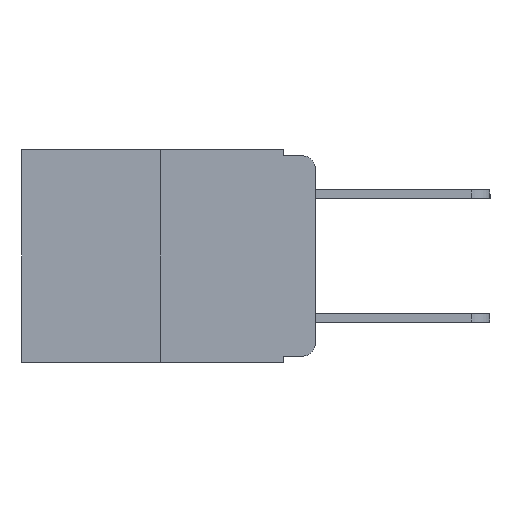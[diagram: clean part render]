
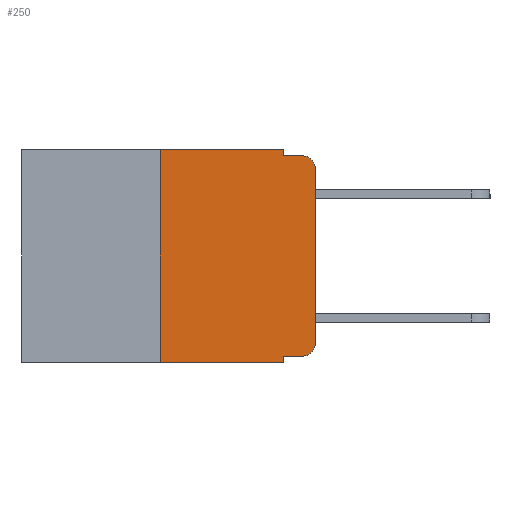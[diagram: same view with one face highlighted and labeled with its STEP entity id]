
A CAD part, left-side view. The second image highlights one B-rep face of the part: STEP entity #250.
In plain terms, the highlighted planar face has unit normal (-1, 0, 0).
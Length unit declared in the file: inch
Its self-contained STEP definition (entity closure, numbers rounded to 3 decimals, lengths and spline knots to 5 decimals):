
#221 = EDGE_CURVE ( 'NONE', #16890, #18291, #3032, .T. ) ;
#250 = ADVANCED_FACE ( 'NONE', ( #1961 ), #18845, .F. ) ;
#632 = EDGE_CURVE ( 'NONE', #7959, #7706, #19525, .T. ) ;
#660 = EDGE_CURVE ( 'NONE', #7706, #18892, #11691, .T. ) ;
#661 = EDGE_CURVE ( 'NONE', #12660, #18892, #18646, .T. ) ;
#666 = EDGE_CURVE ( 'NONE', #18397, #12660, #14743, .T. ) ;
#701 = EDGE_CURVE ( 'NONE', #16890, #14407, #1710, .T. ) ;
#729 = EDGE_CURVE ( 'NONE', #15698, #18291, #13327, .T. ) ;
#741 = EDGE_CURVE ( 'NONE', #15698, #6770, #8849, .T. ) ;
#771 = EDGE_CURVE ( 'NONE', #6770, #7959, #11453, .T. ) ;
#911 = DIRECTION ( 'NONE',  ( 0., 0., 1. ) ) ;
#1091 = CARTESIAN_POINT ( 'NONE',  ( 0., 0.473, 0. ) ) ;
#1710 = LINE ( 'NONE', #16748, #6252 ) ;
#1961 = FACE_OUTER_BOUND ( 'NONE', #14242, .T. ) ;
#2156 = DIRECTION ( 'NONE',  ( 0., -1., 0. ) ) ;
#2264 = DIRECTION ( 'NONE',  ( 0., 0., -1. ) ) ;
#2284 = VECTOR ( 'NONE', #2264, 39.37008 ) ;
#2516 = DIRECTION ( 'NONE',  ( 0., 0., -1. ) ) ;
#2539 = DIRECTION ( 'NONE',  ( 1., 0., 0. ) ) ;
#2591 = CARTESIAN_POINT ( 'NONE',  ( 0., 0.051, -0.01 ) ) ;
#2787 = CARTESIAN_POINT ( 'NONE',  ( 0., 0.051, -0.333 ) ) ;
#3032 = LINE ( 'NONE', #13561, #18817 ) ;
#3086 = ORIENTED_EDGE ( 'NONE', *, *, #10750, .F. ) ;
#3345 = VECTOR ( 'NONE', #10705, 39.37008 ) ;
#4755 = VECTOR ( 'NONE', #17223, 39.37008 ) ;
#4990 = ORIENTED_EDGE ( 'NONE', *, *, #632, .T. ) ;
#5020 = CARTESIAN_POINT ( 'NONE',  ( 0., 0., -0.313 ) ) ;
#6025 = CARTESIAN_POINT ( 'NONE',  ( 0., 0., -0.03 ) ) ;
#6252 = VECTOR ( 'NONE', #911, 39.37008 ) ;
#6271 = CARTESIAN_POINT ( 'NONE',  ( 0., 0., 0. ) ) ;
#6388 = DIRECTION ( 'NONE',  ( -1., 0., 0. ) ) ;
#6457 = CARTESIAN_POINT ( 'NONE',  ( 0., 0.02, -0.03 ) ) ;
#6770 = VERTEX_POINT ( 'NONE', #13465 ) ;
#7179 = ORIENTED_EDGE ( 'NONE', *, *, #661, .F. ) ;
#7253 = ORIENTED_EDGE ( 'NONE', *, *, #660, .T. ) ;
#7706 = VERTEX_POINT ( 'NONE', #6025 ) ;
#7959 = VERTEX_POINT ( 'NONE', #5020 ) ;
#8023 = CARTESIAN_POINT ( 'NONE',  ( 0., 0.02, -0.01 ) ) ;
#8809 = AXIS2_PLACEMENT_3D ( 'NONE', #15366, #15365, #15742 ) ;
#8810 = CARTESIAN_POINT ( 'NONE',  ( 0., 0.051, -0.01 ) ) ;
#8849 = LINE ( 'NONE', #18848, #16406 ) ;
#9087 = ORIENTED_EDGE ( 'NONE', *, *, #666, .F. ) ;
#9106 = CARTESIAN_POINT ( 'NONE',  ( 0., 0.473, 0. ) ) ;
#9413 = DIRECTION ( 'NONE',  ( 0., -1., 0. ) ) ;
#10705 = DIRECTION ( 'NONE',  ( 0., 0., 1. ) ) ;
#10750 = EDGE_CURVE ( 'NONE', #14407, #18397, #18326, .T. ) ;
#10755 = VECTOR ( 'NONE', #9413, 39.37008 ) ;
#10788 = DIRECTION ( 'NONE',  ( 0., -1., 0. ) ) ;
#11453 = CIRCLE ( 'NONE', #8809, 0.02 ) ;
#11486 = CARTESIAN_POINT ( 'NONE',  ( 0., 0.051, 0. ) ) ;
#11691 = CIRCLE ( 'NONE', #17277, 0.02 ) ;
#12348 = ORIENTED_EDGE ( 'NONE', *, *, #221, .T. ) ;
#12568 = ORIENTED_EDGE ( 'NONE', *, *, #701, .F. ) ;
#12660 = VERTEX_POINT ( 'NONE', #8810 ) ;
#13327 = LINE ( 'NONE', #17619, #4755 ) ;
#13465 = CARTESIAN_POINT ( 'NONE',  ( 0., 0.02, -0.333 ) ) ;
#13561 = CARTESIAN_POINT ( 'NONE',  ( 0., 0.473, -0.343 ) ) ;
#13823 = ORIENTED_EDGE ( 'NONE', *, *, #729, .F. ) ;
#14242 = EDGE_LOOP ( 'NONE', ( #4990, #7253, #7179, #9087, #3086, #12568, #12348, #13823, #19174, #18927 ) ) ;
#14351 = VECTOR ( 'NONE', #10788, 39.37008 ) ;
#14407 = VERTEX_POINT ( 'NONE', #15707 ) ;
#14585 = AXIS2_PLACEMENT_3D ( 'NONE', #9106, #2539, #2516 ) ;
#14743 = LINE ( 'NONE', #19656, #2284 ) ;
#15365 = DIRECTION ( 'NONE',  ( -1., 0., 0. ) ) ;
#15366 = CARTESIAN_POINT ( 'NONE',  ( 0., 0.02, -0.313 ) ) ;
#15673 = CARTESIAN_POINT ( 'NONE',  ( 0., 0.051, -0.343 ) ) ;
#15698 = VERTEX_POINT ( 'NONE', #2787 ) ;
#15707 = CARTESIAN_POINT ( 'NONE',  ( 0., 0.25, 0. ) ) ;
#15742 = DIRECTION ( 'NONE',  ( 0., 0., -1. ) ) ;
#16406 = VECTOR ( 'NONE', #17501, 39.37008 ) ;
#16748 = CARTESIAN_POINT ( 'NONE',  ( 0., 0.25, 0. ) ) ;
#16890 = VERTEX_POINT ( 'NONE', #17568 ) ;
#17223 = DIRECTION ( 'NONE',  ( 0., 0., -1. ) ) ;
#17277 = AXIS2_PLACEMENT_3D ( 'NONE', #6457, #6388, #19714 ) ;
#17501 = DIRECTION ( 'NONE',  ( 0., -1., 0. ) ) ;
#17568 = CARTESIAN_POINT ( 'NONE',  ( 0., 0.25, -0.343 ) ) ;
#17619 = CARTESIAN_POINT ( 'NONE',  ( 0., 0.051, 0. ) ) ;
#18291 = VERTEX_POINT ( 'NONE', #15673 ) ;
#18326 = LINE ( 'NONE', #1091, #14351 ) ;
#18397 = VERTEX_POINT ( 'NONE', #11486 ) ;
#18646 = LINE ( 'NONE', #2591, #10755 ) ;
#18817 = VECTOR ( 'NONE', #2156, 39.37008 ) ;
#18845 = PLANE ( 'NONE',  #14585 ) ;
#18848 = CARTESIAN_POINT ( 'NONE',  ( 0., 0.051, -0.333 ) ) ;
#18892 = VERTEX_POINT ( 'NONE', #8023 ) ;
#18927 = ORIENTED_EDGE ( 'NONE', *, *, #771, .T. ) ;
#19174 = ORIENTED_EDGE ( 'NONE', *, *, #741, .T. ) ;
#19525 = LINE ( 'NONE', #6271, #3345 ) ;
#19656 = CARTESIAN_POINT ( 'NONE',  ( 0., 0.051, 0. ) ) ;
#19714 = DIRECTION ( 'NONE',  ( 0., 0., -1. ) ) ;
